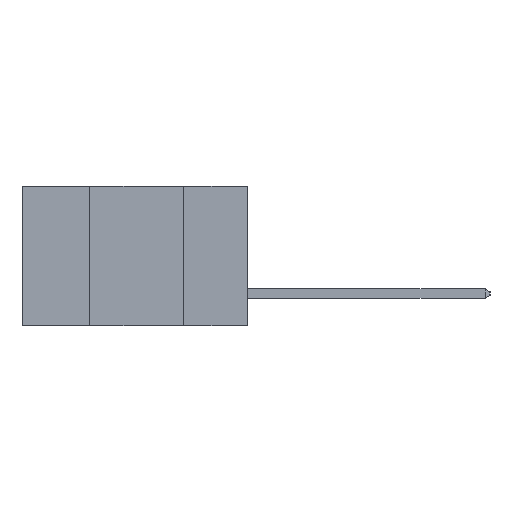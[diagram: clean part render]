
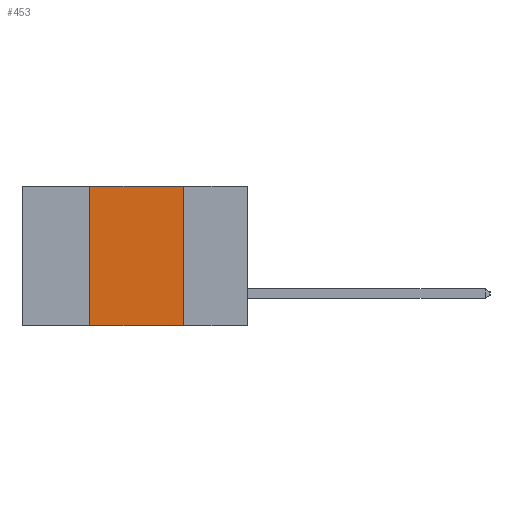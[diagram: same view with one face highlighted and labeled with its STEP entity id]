
A CAD part, left-side view. The second image highlights one B-rep face of the part: STEP entity #453.
In plain terms, the highlighted planar face has unit normal (-1, 0, 0).
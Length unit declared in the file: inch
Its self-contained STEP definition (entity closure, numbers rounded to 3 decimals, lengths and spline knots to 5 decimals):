
#162 = VECTOR ( 'NONE', #11138, 39.37008 ) ;
#380 = ORIENTED_EDGE ( 'NONE', *, *, #6201, .F. ) ;
#453 = ADVANCED_FACE ( 'NONE', ( #17138 ), #5582, .F. ) ;
#505 = ORIENTED_EDGE ( 'NONE', *, *, #1775, .F. ) ;
#650 = EDGE_CURVE ( 'NONE', #7866, #6410, #17377, .T. ) ;
#719 = ORIENTED_EDGE ( 'NONE', *, *, #10479, .F. ) ;
#987 = EDGE_LOOP ( 'NONE', ( #719, #505, #380, #2482 ) ) ;
#1775 = EDGE_CURVE ( 'NONE', #4284, #5294, #5124, .T. ) ;
#1887 = DIRECTION ( 'NONE',  ( 0., 0., 1. ) ) ;
#1892 = CARTESIAN_POINT ( 'NONE',  ( 0., 0.42, 0. ) ) ;
#2482 = ORIENTED_EDGE ( 'NONE', *, *, #650, .T. ) ;
#3631 = DIRECTION ( 'NONE',  ( 0., 0., -1. ) ) ;
#3732 = DIRECTION ( 'NONE',  ( 1., 0., 0. ) ) ;
#4281 = AXIS2_PLACEMENT_3D ( 'NONE', #6726, #3732, #3631 ) ;
#4284 = VERTEX_POINT ( 'NONE', #5115 ) ;
#5115 = CARTESIAN_POINT ( 'NONE',  ( 0., 0.42, 0. ) ) ;
#5124 = LINE ( 'NONE', #11209, #162 ) ;
#5294 = VERTEX_POINT ( 'NONE', #12225 ) ;
#5486 = LINE ( 'NONE', #20294, #13485 ) ;
#5582 = PLANE ( 'NONE',  #4281 ) ;
#6201 = EDGE_CURVE ( 'NONE', #7866, #4284, #18408, .T. ) ;
#6410 = VERTEX_POINT ( 'NONE', #16798 ) ;
#6726 = CARTESIAN_POINT ( 'NONE',  ( 0., 0.6, 0. ) ) ;
#7866 = VERTEX_POINT ( 'NONE', #20562 ) ;
#10479 = EDGE_CURVE ( 'NONE', #5294, #6410, #5486, .T. ) ;
#11138 = DIRECTION ( 'NONE',  ( 0., -1., 0. ) ) ;
#11209 = CARTESIAN_POINT ( 'NONE',  ( 0., 0.6, 0. ) ) ;
#11939 = VECTOR ( 'NONE', #1887, 39.37008 ) ;
#12225 = CARTESIAN_POINT ( 'NONE',  ( 0., 0.17, 0. ) ) ;
#13485 = VECTOR ( 'NONE', #18722, 39.37008 ) ;
#16184 = DIRECTION ( 'NONE',  ( 0., -1., 0. ) ) ;
#16798 = CARTESIAN_POINT ( 'NONE',  ( 0., 0.17, -0.37 ) ) ;
#16875 = VECTOR ( 'NONE', #16184, 39.37008 ) ;
#17138 = FACE_OUTER_BOUND ( 'NONE', #987, .T. ) ;
#17377 = LINE ( 'NONE', #18534, #16875 ) ;
#18408 = LINE ( 'NONE', #1892, #11939 ) ;
#18534 = CARTESIAN_POINT ( 'NONE',  ( 0., 0.6, -0.37 ) ) ;
#18722 = DIRECTION ( 'NONE',  ( 0., 0., -1. ) ) ;
#20294 = CARTESIAN_POINT ( 'NONE',  ( 0., 0.17, 0. ) ) ;
#20562 = CARTESIAN_POINT ( 'NONE',  ( 0., 0.42, -0.37 ) ) ;
